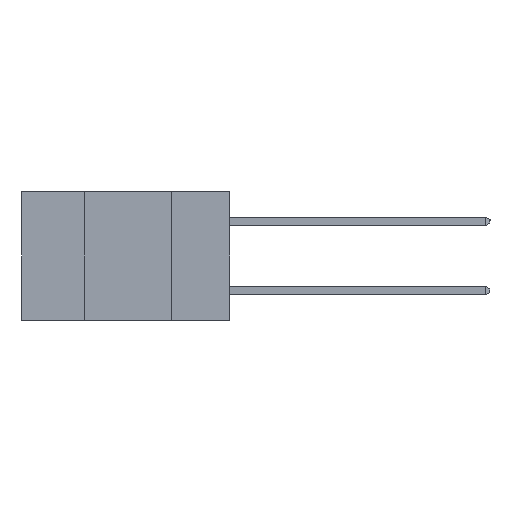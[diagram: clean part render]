
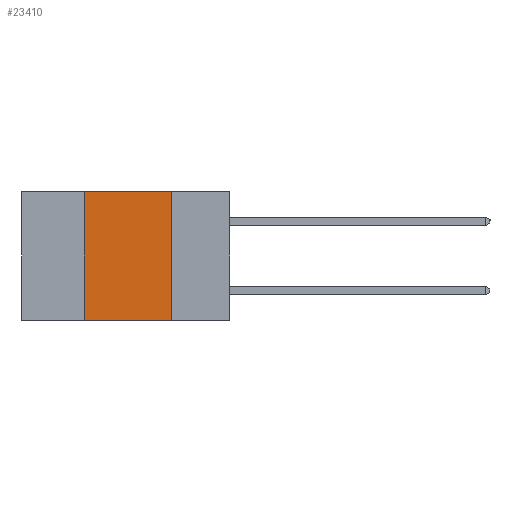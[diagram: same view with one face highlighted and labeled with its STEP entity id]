
A CAD part, left-side view. The second image highlights one B-rep face of the part: STEP entity #23410.
In plain terms, the highlighted planar face has unit normal (-1, 0, 0).
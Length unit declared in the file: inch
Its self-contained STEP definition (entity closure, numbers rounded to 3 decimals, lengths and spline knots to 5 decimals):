
#618 = LINE ( 'NONE', #13764, #19133 ) ;
#873 = AXIS2_PLACEMENT_3D ( 'NONE', #23001, #19532, #10473 ) ;
#1127 = FACE_OUTER_BOUND ( 'NONE', #17931, .T. ) ;
#1676 = CARTESIAN_POINT ( 'NONE',  ( 0., 0.17, -0.37 ) ) ;
#2325 = VERTEX_POINT ( 'NONE', #1676 ) ;
#2973 = CARTESIAN_POINT ( 'NONE',  ( 0., 0.17, 0. ) ) ;
#3763 = VECTOR ( 'NONE', #22913, 39.37008 ) ;
#4234 = VECTOR ( 'NONE', #10192, 39.37008 ) ;
#4445 = VECTOR ( 'NONE', #14571, 39.37008 ) ;
#4461 = EDGE_CURVE ( 'NONE', #18103, #9828, #9433, .T. ) ;
#4763 = CARTESIAN_POINT ( 'NONE',  ( 0., 0.42, -0.37 ) ) ;
#4801 = CARTESIAN_POINT ( 'NONE',  ( 0., 0.17, -0.37 ) ) ;
#5081 = CARTESIAN_POINT ( 'NONE',  ( 0., 0.42, 0. ) ) ;
#8434 = PLANE ( 'NONE',  #873 ) ;
#8586 = EDGE_CURVE ( 'NONE', #20679, #18103, #13964, .T. ) ;
#9433 = LINE ( 'NONE', #10989, #4445 ) ;
#9828 = VERTEX_POINT ( 'NONE', #2973 ) ;
#10192 = DIRECTION ( 'NONE',  ( 0., 0., -1. ) ) ;
#10473 = DIRECTION ( 'NONE',  ( 0., 0., -1. ) ) ;
#10989 = CARTESIAN_POINT ( 'NONE',  ( 0., 0.6, 0. ) ) ;
#12444 = EDGE_CURVE ( 'NONE', #9828, #2325, #19244, .T. ) ;
#13362 = ORIENTED_EDGE ( 'NONE', *, *, #12444, .F. ) ;
#13648 = DIRECTION ( 'NONE',  ( 0., -1., 0. ) ) ;
#13764 = CARTESIAN_POINT ( 'NONE',  ( 0., 0.6, -0.37 ) ) ;
#13964 = LINE ( 'NONE', #4763, #3763 ) ;
#14571 = DIRECTION ( 'NONE',  ( 0., -1., 0. ) ) ;
#17135 = CARTESIAN_POINT ( 'NONE',  ( 0., 0.42, -0.37 ) ) ;
#17931 = EDGE_LOOP ( 'NONE', ( #13362, #18283, #21337, #19102 ) ) ;
#18103 = VERTEX_POINT ( 'NONE', #5081 ) ;
#18283 = ORIENTED_EDGE ( 'NONE', *, *, #4461, .F. ) ;
#19102 = ORIENTED_EDGE ( 'NONE', *, *, #22385, .T. ) ;
#19133 = VECTOR ( 'NONE', #13648, 39.37008 ) ;
#19244 = LINE ( 'NONE', #4801, #4234 ) ;
#19532 = DIRECTION ( 'NONE',  ( 1., 0., 0. ) ) ;
#20679 = VERTEX_POINT ( 'NONE', #17135 ) ;
#21337 = ORIENTED_EDGE ( 'NONE', *, *, #8586, .F. ) ;
#22385 = EDGE_CURVE ( 'NONE', #20679, #2325, #618, .T. ) ;
#22913 = DIRECTION ( 'NONE',  ( 0., 0., 1. ) ) ;
#23001 = CARTESIAN_POINT ( 'NONE',  ( 0., 0.6, 0. ) ) ;
#23410 = ADVANCED_FACE ( 'NONE', ( #1127 ), #8434, .F. ) ;
